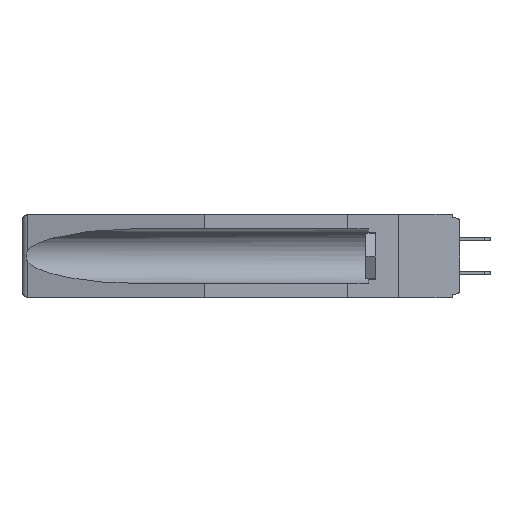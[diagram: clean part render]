
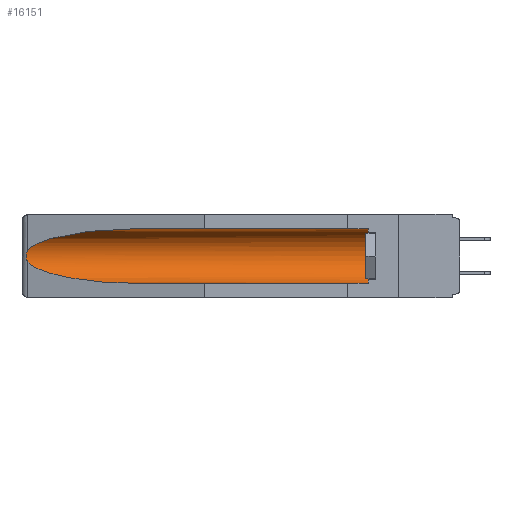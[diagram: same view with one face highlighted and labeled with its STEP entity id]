
A CAD part, left-side view. The second image highlights one B-rep face of the part: STEP entity #16151.
In plain terms, the highlighted cylindrical face has radius 2.857 mm (diameter 5.715 mm), a partial arc.
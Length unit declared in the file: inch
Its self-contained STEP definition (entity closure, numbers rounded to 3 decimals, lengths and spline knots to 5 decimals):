
#349 = CARTESIAN_POINT ( 'NONE',  ( 0.26537, 1.52718, -0.19328 ) ) ;
#502 = B_SPLINE_CURVE_WITH_KNOTS ( 'NONE', 3,
 ( #14393, #17360, #2231, #11235, #18974, #11309, #12847, #4406, #6090, #9207 ),
 .UNSPECIFIED., .F., .F.,
 ( 4, 2, 2, 2, 4 ),
 ( 0., 0.00029, 0.00058, 0.00087, 0.00117 ),
 .UNSPECIFIED. ) ;
#652 = LINE ( 'NONE', #3846, #16537 ) ;
#972 = CARTESIAN_POINT ( 'NONE',  ( 0.155, 0.126, -0.059 ) ) ;
#998 = VECTOR ( 'NONE', #14831, 39.37008 ) ;
#2231 = CARTESIAN_POINT ( 'NONE',  ( 0.26654, 1.53092, -0.15636 ) ) ;
#3317 = CARTESIAN_POINT ( 'NONE',  ( 0.25451, 1.48313, -0.24835 ) ) ;
#3479 = CIRCLE ( 'NONE', #9418, 0.1125 ) ;
#3513 = CARTESIAN_POINT ( 'NONE',  ( 0.155, -0.30754, -0.1715 ) ) ;
#3846 = CARTESIAN_POINT ( 'NONE',  ( 0.155, -0.30754, -0.059 ) ) ;
#3934 = EDGE_CURVE ( 'NONE', #4501, #17053, #502, .T. ) ;
#4372 = VERTEX_POINT ( 'NONE', #17430 ) ;
#4406 = CARTESIAN_POINT ( 'NONE',  ( 0.26655, 1.53094, -0.18657 ) ) ;
#4462 = CARTESIAN_POINT ( 'NONE',  ( 0.26537, 1.52718, -0.19328 ) ) ;
#4501 = VERTEX_POINT ( 'NONE', #18472 ) ;
#4607 = DIRECTION ( 'NONE',  ( 0., -1., 0. ) ) ;
#5922 = ORIENTED_EDGE ( 'NONE', *, *, #17931, .T. ) ;
#6090 = CARTESIAN_POINT ( 'NONE',  ( 0.26597, 1.5296, -0.19026 ) ) ;
#6191 =( BOUNDED_CURVE ( )  B_SPLINE_CURVE ( 3, ( #4462, #3317, #6404, #14209 ),
 .UNSPECIFIED., .F., .F. ) 
 B_SPLINE_CURVE_WITH_KNOTS ( ( 4, 4 ),
 ( 0.1948, 1.5708 ),
 .UNSPECIFIED. ) 
 CURVE ( )  GEOMETRIC_REPRESENTATION_ITEM ( )  RATIONAL_B_SPLINE_CURVE ( ( 1., 0.848, 0.848, 1. ) ) 
 REPRESENTATION_ITEM ( '' )  );
#6404 = CARTESIAN_POINT ( 'NONE',  ( 0.21114, 1.30732, -0.284 ) ) ;
#6535 = DIRECTION ( 'NONE',  ( 0., 1., 0. ) ) ;
#7071 = ORIENTED_EDGE ( 'NONE', *, *, #15016, .F. ) ;
#7154 = EDGE_CURVE ( 'NONE', #4372, #4501, #9796, .T. ) ;
#7262 = CARTESIAN_POINT ( 'NONE',  ( 0.155, 1.07973, -0.059 ) ) ;
#7816 = EDGE_CURVE ( 'NONE', #16313, #4372, #652, .T. ) ;
#8682 = FACE_OUTER_BOUND ( 'NONE', #15638, .T. ) ;
#8890 = EDGE_CURVE ( 'NONE', #17053, #15489, #6191, .T. ) ;
#9174 = CYLINDRICAL_SURFACE ( 'NONE', #17331, 0.1125 ) ;
#9205 = CARTESIAN_POINT ( 'NONE',  ( 0.25451, 1.48313, -0.09465 ) ) ;
#9207 = CARTESIAN_POINT ( 'NONE',  ( 0.26537, 1.52718, -0.19328 ) ) ;
#9418 = AXIS2_PLACEMENT_3D ( 'NONE', #13811, #4607, #18328 ) ;
#9560 = CARTESIAN_POINT ( 'NONE',  ( 0.155, 1.07973, -0.284 ) ) ;
#9796 =( BOUNDED_CURVE ( )  B_SPLINE_CURVE ( 3, ( #7262, #19596, #9205, #10470 ),
 .UNSPECIFIED., .F., .F. ) 
 B_SPLINE_CURVE_WITH_KNOTS ( ( 4, 4 ),
 ( 4.71239, 6.08839 ),
 .UNSPECIFIED. ) 
 CURVE ( )  GEOMETRIC_REPRESENTATION_ITEM ( )  RATIONAL_B_SPLINE_CURVE ( ( 1., 0.848, 0.848, 1. ) ) 
 REPRESENTATION_ITEM ( '' )  );
#10320 = VERTEX_POINT ( 'NONE', #15422 ) ;
#10470 = CARTESIAN_POINT ( 'NONE',  ( 0.26537, 1.52718, -0.14972 ) ) ;
#11099 = DIRECTION ( 'NONE',  ( 0., 0., 1. ) ) ;
#11235 = CARTESIAN_POINT ( 'NONE',  ( 0.2673, 1.5327, -0.16383 ) ) ;
#11309 = CARTESIAN_POINT ( 'NONE',  ( 0.2675, 1.53308, -0.17534 ) ) ;
#11491 = CARTESIAN_POINT ( 'NONE',  ( 0.155, -0.30754, -0.284 ) ) ;
#11548 = ORIENTED_EDGE ( 'NONE', *, *, #7816, .T. ) ;
#12847 = CARTESIAN_POINT ( 'NONE',  ( 0.2673, 1.53269, -0.17917 ) ) ;
#13811 = CARTESIAN_POINT ( 'NONE',  ( 0.155, 0.126, -0.1715 ) ) ;
#14209 = CARTESIAN_POINT ( 'NONE',  ( 0.155, 1.07973, -0.284 ) ) ;
#14393 = CARTESIAN_POINT ( 'NONE',  ( 0.26537, 1.52718, -0.14972 ) ) ;
#14831 = DIRECTION ( 'NONE',  ( 0., 1., 0. ) ) ;
#14992 = ORIENTED_EDGE ( 'NONE', *, *, #8890, .T. ) ;
#15016 = EDGE_CURVE ( 'NONE', #10320, #15489, #17887, .T. ) ;
#15422 = CARTESIAN_POINT ( 'NONE',  ( 0.155, 0.126, -0.284 ) ) ;
#15489 = VERTEX_POINT ( 'NONE', #9560 ) ;
#15638 = EDGE_LOOP ( 'NONE', ( #16411, #18633, #14992, #7071, #5922, #11548 ) ) ;
#16151 = ADVANCED_FACE ( 'NONE', ( #8682 ), #9174, .F. ) ;
#16313 = VERTEX_POINT ( 'NONE', #972 ) ;
#16411 = ORIENTED_EDGE ( 'NONE', *, *, #7154, .T. ) ;
#16537 = VECTOR ( 'NONE', #17570, 39.37008 ) ;
#17053 = VERTEX_POINT ( 'NONE', #349 ) ;
#17331 = AXIS2_PLACEMENT_3D ( 'NONE', #3513, #6535, #11099 ) ;
#17360 = CARTESIAN_POINT ( 'NONE',  ( 0.26597, 1.52961, -0.15275 ) ) ;
#17430 = CARTESIAN_POINT ( 'NONE',  ( 0.155, 1.07973, -0.059 ) ) ;
#17570 = DIRECTION ( 'NONE',  ( 0., 1., 0. ) ) ;
#17887 = LINE ( 'NONE', #11491, #998 ) ;
#17931 = EDGE_CURVE ( 'NONE', #10320, #16313, #3479, .T. ) ;
#18328 = DIRECTION ( 'NONE',  ( 0., 0., 1. ) ) ;
#18472 = CARTESIAN_POINT ( 'NONE',  ( 0.26537, 1.52718, -0.14972 ) ) ;
#18633 = ORIENTED_EDGE ( 'NONE', *, *, #3934, .T. ) ;
#18974 = CARTESIAN_POINT ( 'NONE',  ( 0.2675, 1.53308, -0.16763 ) ) ;
#19596 = CARTESIAN_POINT ( 'NONE',  ( 0.21114, 1.30732, -0.059 ) ) ;
